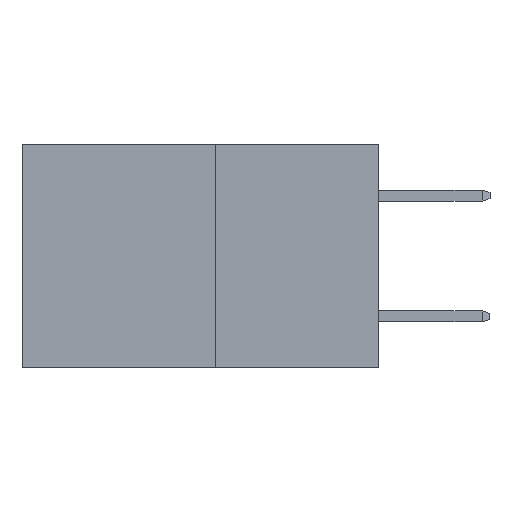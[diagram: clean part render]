
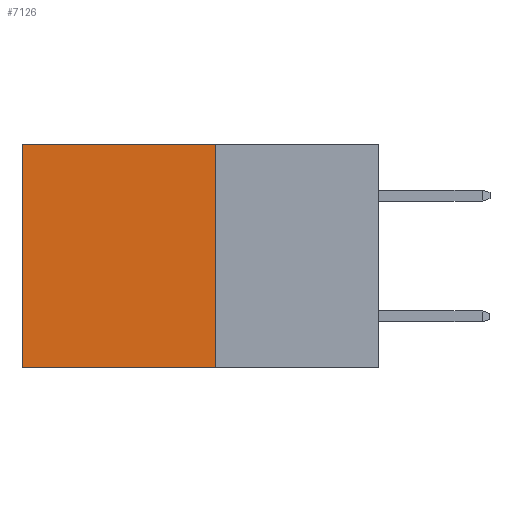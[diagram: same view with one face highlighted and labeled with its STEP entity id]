
A CAD part, left-side view. The second image highlights one B-rep face of the part: STEP entity #7126.
In plain terms, the highlighted planar face has unit normal (-1, 0, 0).
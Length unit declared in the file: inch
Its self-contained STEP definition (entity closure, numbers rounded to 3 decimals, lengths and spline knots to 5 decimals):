
#69 = EDGE_CURVE ( 'NONE', #1012, #1973, #7576, .T. ) ;
#177 = VERTEX_POINT ( 'NONE', #6829 ) ;
#389 = VERTEX_POINT ( 'NONE', #4301 ) ;
#472 = EDGE_CURVE ( 'NONE', #1012, #389, #6404, .T. ) ;
#690 = DIRECTION ( 'NONE',  ( 1., 0., 0. ) ) ;
#1012 = VERTEX_POINT ( 'NONE', #7197 ) ;
#1093 = EDGE_LOOP ( 'NONE', ( #7594, #2067, #3694, #6508 ) ) ;
#1165 = CARTESIAN_POINT ( 'NONE',  ( 0.277, 0.59, -0.37 ) ) ;
#1335 = VECTOR ( 'NONE', #3379, 39.37008 ) ;
#1610 = VECTOR ( 'NONE', #5287, 39.37008 ) ;
#1831 = LINE ( 'NONE', #3303, #1610 ) ;
#1973 = VERTEX_POINT ( 'NONE', #3573 ) ;
#2067 = ORIENTED_EDGE ( 'NONE', *, *, #5485, .F. ) ;
#2851 = EDGE_CURVE ( 'NONE', #1973, #177, #6012, .T. ) ;
#3098 = DIRECTION ( 'NONE',  ( 0., 1., 0. ) ) ;
#3303 = CARTESIAN_POINT ( 'NONE',  ( 0.277, 0.27, -0.37 ) ) ;
#3379 = DIRECTION ( 'NONE',  ( 0., 0., -1. ) ) ;
#3503 = VECTOR ( 'NONE', #4217, 39.37008 ) ;
#3573 = CARTESIAN_POINT ( 'NONE',  ( 0.277, 0.59, 0. ) ) ;
#3694 = ORIENTED_EDGE ( 'NONE', *, *, #472, .F. ) ;
#4217 = DIRECTION ( 'NONE',  ( 0., 0., -1. ) ) ;
#4301 = CARTESIAN_POINT ( 'NONE',  ( 0.277, 0.27, -0.37 ) ) ;
#4313 = AXIS2_PLACEMENT_3D ( 'NONE', #4826, #690, #4523 ) ;
#4523 = DIRECTION ( 'NONE',  ( 0., 0., -1. ) ) ;
#4826 = CARTESIAN_POINT ( 'NONE',  ( 0.277, 0.27, -0.37 ) ) ;
#5287 = DIRECTION ( 'NONE',  ( 0., 1., 0. ) ) ;
#5485 = EDGE_CURVE ( 'NONE', #389, #177, #1831, .T. ) ;
#5658 = FACE_OUTER_BOUND ( 'NONE', #1093, .T. ) ;
#6012 = LINE ( 'NONE', #1165, #1335 ) ;
#6054 = VECTOR ( 'NONE', #3098, 39.37008 ) ;
#6404 = LINE ( 'NONE', #7452, #3503 ) ;
#6508 = ORIENTED_EDGE ( 'NONE', *, *, #69, .T. ) ;
#6702 = PLANE ( 'NONE',  #4313 ) ;
#6721 = CARTESIAN_POINT ( 'NONE',  ( 0.277, 0.27, 0. ) ) ;
#6829 = CARTESIAN_POINT ( 'NONE',  ( 0.277, 0.59, -0.37 ) ) ;
#7126 = ADVANCED_FACE ( 'NONE', ( #5658 ), #6702, .F. ) ;
#7197 = CARTESIAN_POINT ( 'NONE',  ( 0.277, 0.27, 0. ) ) ;
#7452 = CARTESIAN_POINT ( 'NONE',  ( 0.277, 0.27, -0.37 ) ) ;
#7576 = LINE ( 'NONE', #6721, #6054 ) ;
#7594 = ORIENTED_EDGE ( 'NONE', *, *, #2851, .T. ) ;
